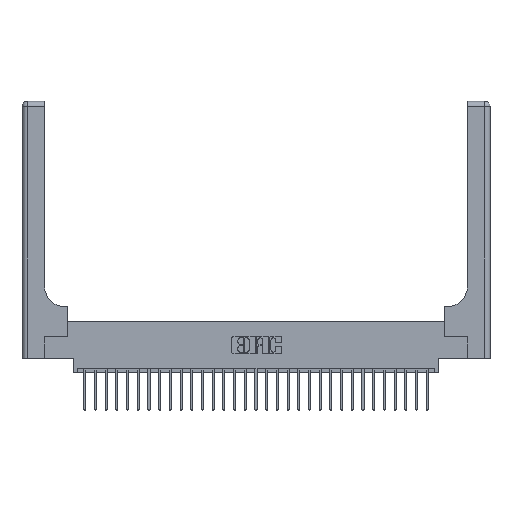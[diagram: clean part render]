
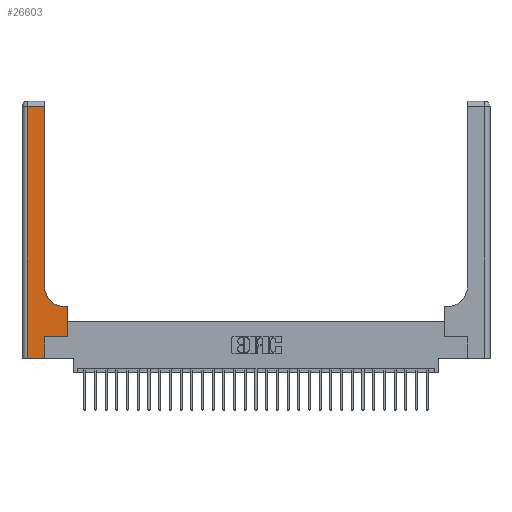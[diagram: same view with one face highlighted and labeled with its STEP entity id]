
A CAD part, top view. The second image highlights one B-rep face of the part: STEP entity #26603.
In plain terms, the highlighted planar face has unit normal (0, 0, 1).
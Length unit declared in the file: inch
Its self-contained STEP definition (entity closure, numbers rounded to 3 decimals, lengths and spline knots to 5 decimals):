
#158 = EDGE_CURVE ( 'NONE', #10084, #13579, #16594, .T. ) ;
#515 = EDGE_CURVE ( 'NONE', #16744, #6418, #19925, .T. ) ;
#566 = LINE ( 'NONE', #8530, #27364 ) ;
#1613 = CARTESIAN_POINT ( 'NONE',  ( 0.265, 0., 0.37 ) ) ;
#1726 = DIRECTION ( 'NONE',  ( 0., 1., 0. ) ) ;
#1742 = ORIENTED_EDGE ( 'NONE', *, *, #24238, .T. ) ;
#1769 = ORIENTED_EDGE ( 'NONE', *, *, #27217, .T. ) ;
#1779 = CARTESIAN_POINT ( 'NONE',  ( 0.51, 0.85, 0.37 ) ) ;
#2129 = VERTEX_POINT ( 'NONE', #18465 ) ;
#2232 = VERTEX_POINT ( 'NONE', #14656 ) ;
#3006 = VERTEX_POINT ( 'NONE', #3626 ) ;
#3626 = CARTESIAN_POINT ( 'NONE',  ( 0.06, 0., 0.37 ) ) ;
#3664 = FACE_OUTER_BOUND ( 'NONE', #26361, .T. ) ;
#3969 = DIRECTION ( 'NONE',  ( 1., 0., 0. ) ) ;
#4065 = CIRCLE ( 'NONE', #4086, 0.25 ) ;
#4086 = AXIS2_PLACEMENT_3D ( 'NONE', #1779, #17073, #3969 ) ;
#4298 = PLANE ( 'NONE',  #10285 ) ;
#4408 = CARTESIAN_POINT ( 'NONE',  ( 0.265, 0.25, 0.37 ) ) ;
#4410 = EDGE_CURVE ( 'NONE', #2129, #16744, #566, .T. ) ;
#4744 = CARTESIAN_POINT ( 'NONE',  ( 0., 0., 0.37 ) ) ;
#5682 = ORIENTED_EDGE ( 'NONE', *, *, #9692, .T. ) ;
#6418 = VERTEX_POINT ( 'NONE', #9773 ) ;
#6499 = DIRECTION ( 'NONE',  ( 0., 0., -1. ) ) ;
#6854 = CARTESIAN_POINT ( 'NONE',  ( 0.06, 3., 0.37 ) ) ;
#7050 = ORIENTED_EDGE ( 'NONE', *, *, #515, .T. ) ;
#8112 = CARTESIAN_POINT ( 'NONE',  ( 0.265, 0.25, 0.37 ) ) ;
#8306 = CARTESIAN_POINT ( 'NONE',  ( 0.528, 0.25, 0.37 ) ) ;
#8530 = CARTESIAN_POINT ( 'NONE',  ( 0.26, 3., 0.37 ) ) ;
#9014 = DIRECTION ( 'NONE',  ( 0., -1., 0. ) ) ;
#9692 = EDGE_CURVE ( 'NONE', #25226, #10084, #21302, .T. ) ;
#9773 = CARTESIAN_POINT ( 'NONE',  ( 0.06, 2.94, 0.37 ) ) ;
#10084 = VERTEX_POINT ( 'NONE', #8112 ) ;
#10285 = AXIS2_PLACEMENT_3D ( 'NONE', #19517, #6499, #21678 ) ;
#10441 = VECTOR ( 'NONE', #9014, 39.37008 ) ;
#12122 = CARTESIAN_POINT ( 'NONE',  ( 0.26, 2.94, 0.37 ) ) ;
#12422 = DIRECTION ( 'NONE',  ( -1., 0., 0. ) ) ;
#13579 = VERTEX_POINT ( 'NONE', #22867 ) ;
#14135 = VECTOR ( 'NONE', #12422, 39.37008 ) ;
#14604 = VERTEX_POINT ( 'NONE', #16111 ) ;
#14656 = CARTESIAN_POINT ( 'NONE',  ( 0.528, 0.6, 0.37 ) ) ;
#14711 = VECTOR ( 'NONE', #24284, 39.37008 ) ;
#15245 = ORIENTED_EDGE ( 'NONE', *, *, #158, .T. ) ;
#15706 = DIRECTION ( 'NONE',  ( -1., 0., 0. ) ) ;
#15802 = CARTESIAN_POINT ( 'NONE',  ( 0.26, 0.6, 0.37 ) ) ;
#16111 = CARTESIAN_POINT ( 'NONE',  ( 0.51, 0.6, 0.37 ) ) ;
#16594 = LINE ( 'NONE', #4408, #21635 ) ;
#16704 = VECTOR ( 'NONE', #15706, 39.37008 ) ;
#16744 = VERTEX_POINT ( 'NONE', #12122 ) ;
#16877 = LINE ( 'NONE', #8306, #23255 ) ;
#17073 = DIRECTION ( 'NONE',  ( 0., 0., -1. ) ) ;
#18465 = CARTESIAN_POINT ( 'NONE',  ( 0.26, 0.85, 0.37 ) ) ;
#18808 = EDGE_CURVE ( 'NONE', #2232, #14604, #22417, .T. ) ;
#19517 = CARTESIAN_POINT ( 'NONE',  ( 0., 3., 0.37 ) ) ;
#19921 = DIRECTION ( 'NONE',  ( 0., 1., 0. ) ) ;
#19925 = LINE ( 'NONE', #23274, #14135 ) ;
#20164 = ORIENTED_EDGE ( 'NONE', *, *, #21880, .T. ) ;
#21164 = LINE ( 'NONE', #4744, #14711 ) ;
#21302 = LINE ( 'NONE', #24167, #25631 ) ;
#21635 = VECTOR ( 'NONE', #23962, 39.37008 ) ;
#21678 = DIRECTION ( 'NONE',  ( -1., 0., 0. ) ) ;
#21880 = EDGE_CURVE ( 'NONE', #13579, #2232, #16877, .T. ) ;
#22417 = LINE ( 'NONE', #15802, #16704 ) ;
#22867 = CARTESIAN_POINT ( 'NONE',  ( 0.528, 0.25, 0.37 ) ) ;
#23255 = VECTOR ( 'NONE', #1726, 39.37008 ) ;
#23274 = CARTESIAN_POINT ( 'NONE',  ( 0., 2.94, 0.37 ) ) ;
#23962 = DIRECTION ( 'NONE',  ( 1., 0., 0. ) ) ;
#24167 = CARTESIAN_POINT ( 'NONE',  ( 0.265, 0., 0.37 ) ) ;
#24238 = EDGE_CURVE ( 'NONE', #3006, #25226, #21164, .T. ) ;
#24284 = DIRECTION ( 'NONE',  ( 1., 0., 0. ) ) ;
#25089 = ORIENTED_EDGE ( 'NONE', *, *, #25811, .T. ) ;
#25177 = ORIENTED_EDGE ( 'NONE', *, *, #4410, .T. ) ;
#25226 = VERTEX_POINT ( 'NONE', #1613 ) ;
#25631 = VECTOR ( 'NONE', #19921, 39.37008 ) ;
#25811 = EDGE_CURVE ( 'NONE', #14604, #2129, #4065, .T. ) ;
#26361 = EDGE_LOOP ( 'NONE', ( #25177, #7050, #1769, #1742, #5682, #15245, #20164, #27012, #25089 ) ) ;
#26603 = ADVANCED_FACE ( 'NONE', ( #3664 ), #4298, .F. ) ;
#27012 = ORIENTED_EDGE ( 'NONE', *, *, #18808, .T. ) ;
#27217 = EDGE_CURVE ( 'NONE', #6418, #3006, #27674, .T. ) ;
#27364 = VECTOR ( 'NONE', #27969, 39.37008 ) ;
#27674 = LINE ( 'NONE', #6854, #10441 ) ;
#27969 = DIRECTION ( 'NONE',  ( 0., 1., 0. ) ) ;
